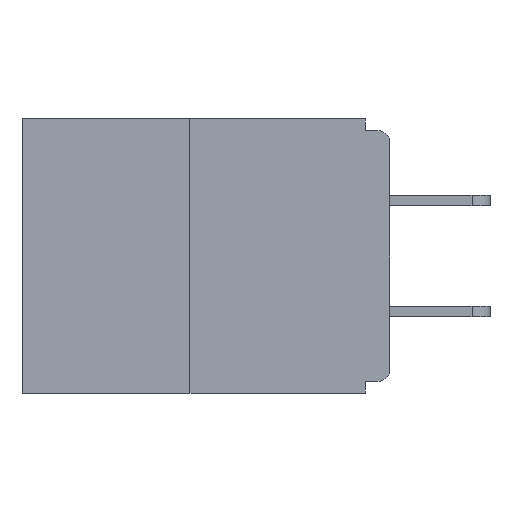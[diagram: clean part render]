
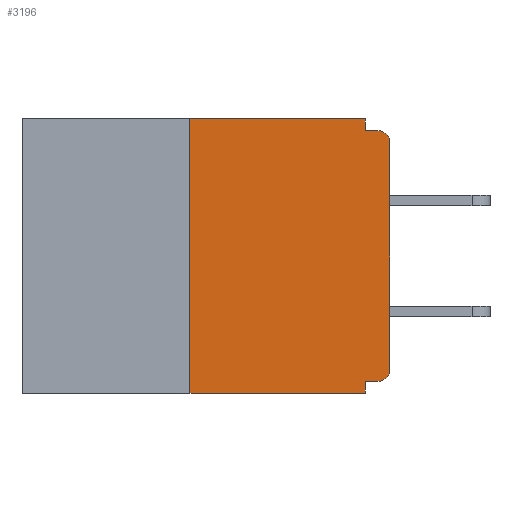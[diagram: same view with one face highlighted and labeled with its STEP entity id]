
A CAD part, left-side view. The second image highlights one B-rep face of the part: STEP entity #3196.
In plain terms, the highlighted planar face has unit normal (-1, 0, 0).
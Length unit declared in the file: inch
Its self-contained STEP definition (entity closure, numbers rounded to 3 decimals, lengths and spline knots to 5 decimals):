
#160 = EDGE_CURVE ( 'NONE', #17063, #9064, #20758, .T. ) ;
#390 = LINE ( 'NONE', #18195, #13068 ) ;
#775 = ORIENTED_EDGE ( 'NONE', *, *, #22929, .T. ) ;
#793 = CARTESIAN_POINT ( 'NONE',  ( 0., 0.031, -0.015 ) ) ;
#862 = ORIENTED_EDGE ( 'NONE', *, *, #13234, .F. ) ;
#1374 = ORIENTED_EDGE ( 'NONE', *, *, #11566, .F. ) ;
#1934 = DIRECTION ( 'NONE',  ( 0., 0., 1. ) ) ;
#2042 = EDGE_CURVE ( 'NONE', #4062, #8359, #8347, .T. ) ;
#2133 = ORIENTED_EDGE ( 'NONE', *, *, #2042, .F. ) ;
#2252 = ORIENTED_EDGE ( 'NONE', *, *, #21630, .F. ) ;
#2336 = VECTOR ( 'NONE', #8864, 39.37008 ) ;
#2430 = DIRECTION ( 'NONE',  ( 0., 0., -1. ) ) ;
#2885 = CARTESIAN_POINT ( 'NONE',  ( 0., 0.46, 0. ) ) ;
#2946 = AXIS2_PLACEMENT_3D ( 'NONE', #19998, #8710, #12509 ) ;
#3078 = DIRECTION ( 'NONE',  ( 0., 0., 1. ) ) ;
#3196 = ADVANCED_FACE ( 'NONE', ( #16553 ), #7989, .F. ) ;
#3517 = LINE ( 'NONE', #12507, #2336 ) ;
#3755 = CARTESIAN_POINT ( 'NONE',  ( 0., 0.031, -0.343 ) ) ;
#3769 = LINE ( 'NONE', #13765, #11201 ) ;
#4062 = VERTEX_POINT ( 'NONE', #4425 ) ;
#4416 = DIRECTION ( 'NONE',  ( -1., 0., 0. ) ) ;
#4425 = CARTESIAN_POINT ( 'NONE',  ( 0., 0.031, -0.328 ) ) ;
#4554 = ORIENTED_EDGE ( 'NONE', *, *, #17273, .T. ) ;
#4555 = LINE ( 'NONE', #21785, #12803 ) ;
#4602 = VECTOR ( 'NONE', #1934, 39.37008 ) ;
#4649 = VERTEX_POINT ( 'NONE', #14030 ) ;
#4992 = CARTESIAN_POINT ( 'NONE',  ( 0., 0.25, 0. ) ) ;
#5268 = EDGE_LOOP ( 'NONE', ( #19015, #12070, #18105, #2133, #862, #19590, #775, #4554, #2252, #1374 ) ) ;
#5684 = VECTOR ( 'NONE', #16126, 39.37008 ) ;
#6027 = CARTESIAN_POINT ( 'NONE',  ( 0., 0.46, 0. ) ) ;
#6042 = CARTESIAN_POINT ( 'NONE',  ( 0., 0., -0.328 ) ) ;
#6323 = EDGE_CURVE ( 'NONE', #9884, #10009, #14652, .T. ) ;
#6984 = LINE ( 'NONE', #6042, #17611 ) ;
#7150 = CARTESIAN_POINT ( 'NONE',  ( 0., 0.015, -0.328 ) ) ;
#7181 = VERTEX_POINT ( 'NONE', #793 ) ;
#7507 = DIRECTION ( 'NONE',  ( 0., 0., -1. ) ) ;
#7989 = PLANE ( 'NONE',  #19402 ) ;
#8347 = LINE ( 'NONE', #3755, #11306 ) ;
#8359 = VERTEX_POINT ( 'NONE', #22632 ) ;
#8710 = DIRECTION ( 'NONE',  ( -1., 0., 0. ) ) ;
#8864 = DIRECTION ( 'NONE',  ( 0., -1., 0. ) ) ;
#9064 = VERTEX_POINT ( 'NONE', #10152 ) ;
#9884 = VERTEX_POINT ( 'NONE', #21348 ) ;
#9973 = DIRECTION ( 'NONE',  ( 0., 1., 0. ) ) ;
#10009 = VERTEX_POINT ( 'NONE', #4992 ) ;
#10042 = VERTEX_POINT ( 'NONE', #10705 ) ;
#10152 = CARTESIAN_POINT ( 'NONE',  ( 0., 0., -0.313 ) ) ;
#10705 = CARTESIAN_POINT ( 'NONE',  ( 0., 0.015, -0.015 ) ) ;
#11201 = VECTOR ( 'NONE', #2430, 39.37008 ) ;
#11306 = VECTOR ( 'NONE', #7507, 39.37008 ) ;
#11388 = CARTESIAN_POINT ( 'NONE',  ( 0., 0.25, 0. ) ) ;
#11566 = EDGE_CURVE ( 'NONE', #4649, #7181, #3769, .T. ) ;
#11712 = CARTESIAN_POINT ( 'NONE',  ( 0., 0.015, -0.313 ) ) ;
#12070 = ORIENTED_EDGE ( 'NONE', *, *, #6323, .F. ) ;
#12507 = CARTESIAN_POINT ( 'NONE',  ( 0., 0.46, -0.343 ) ) ;
#12509 = DIRECTION ( 'NONE',  ( 0., 0., -1. ) ) ;
#12540 = DIRECTION ( 'NONE',  ( 0., -1., 0. ) ) ;
#12803 = VECTOR ( 'NONE', #12540, 39.37008 ) ;
#13068 = VECTOR ( 'NONE', #3078, 39.37008 ) ;
#13234 = EDGE_CURVE ( 'NONE', #17063, #4062, #6984, .T. ) ;
#13765 = CARTESIAN_POINT ( 'NONE',  ( 0., 0.031, 0. ) ) ;
#14030 = CARTESIAN_POINT ( 'NONE',  ( 0., 0.031, 0. ) ) ;
#14216 = LINE ( 'NONE', #2885, #5684 ) ;
#14652 = LINE ( 'NONE', #11388, #4602 ) ;
#15234 = DIRECTION ( 'NONE',  ( 1., 0., 0. ) ) ;
#16126 = DIRECTION ( 'NONE',  ( 0., -1., 0. ) ) ;
#16553 = FACE_OUTER_BOUND ( 'NONE', #5268, .T. ) ;
#17063 = VERTEX_POINT ( 'NONE', #7150 ) ;
#17273 = EDGE_CURVE ( 'NONE', #19788, #10042, #18500, .T. ) ;
#17611 = VECTOR ( 'NONE', #9973, 39.37008 ) ;
#17616 = DIRECTION ( 'NONE',  ( 0., 0., -1. ) ) ;
#18105 = ORIENTED_EDGE ( 'NONE', *, *, #18276, .T. ) ;
#18195 = CARTESIAN_POINT ( 'NONE',  ( 0., 0., 0. ) ) ;
#18276 = EDGE_CURVE ( 'NONE', #9884, #8359, #3517, .T. ) ;
#18500 = CIRCLE ( 'NONE', #2946, 0.015 ) ;
#19015 = ORIENTED_EDGE ( 'NONE', *, *, #23436, .F. ) ;
#19402 = AXIS2_PLACEMENT_3D ( 'NONE', #6027, #15234, #22666 ) ;
#19590 = ORIENTED_EDGE ( 'NONE', *, *, #160, .T. ) ;
#19788 = VERTEX_POINT ( 'NONE', #23762 ) ;
#19998 = CARTESIAN_POINT ( 'NONE',  ( 0., 0.015, -0.03 ) ) ;
#20758 = CIRCLE ( 'NONE', #24255, 0.015 ) ;
#21348 = CARTESIAN_POINT ( 'NONE',  ( 0., 0.25, -0.343 ) ) ;
#21630 = EDGE_CURVE ( 'NONE', #7181, #10042, #4555, .T. ) ;
#21785 = CARTESIAN_POINT ( 'NONE',  ( 0., 0., -0.015 ) ) ;
#22632 = CARTESIAN_POINT ( 'NONE',  ( 0., 0.031, -0.343 ) ) ;
#22666 = DIRECTION ( 'NONE',  ( 0., 0., -1. ) ) ;
#22929 = EDGE_CURVE ( 'NONE', #9064, #19788, #390, .T. ) ;
#23436 = EDGE_CURVE ( 'NONE', #10009, #4649, #14216, .T. ) ;
#23762 = CARTESIAN_POINT ( 'NONE',  ( 0., 0., -0.03 ) ) ;
#24255 = AXIS2_PLACEMENT_3D ( 'NONE', #11712, #4416, #17616 ) ;
